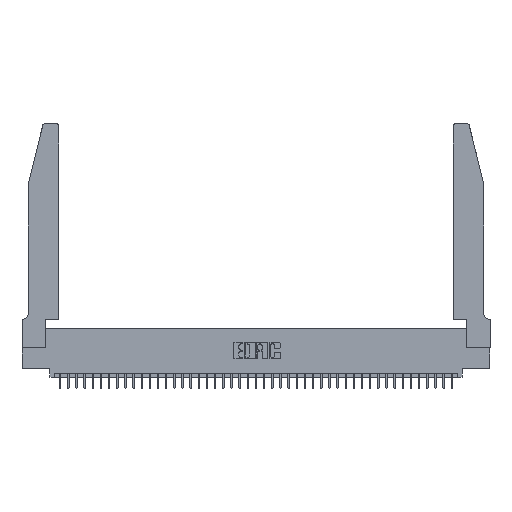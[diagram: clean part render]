
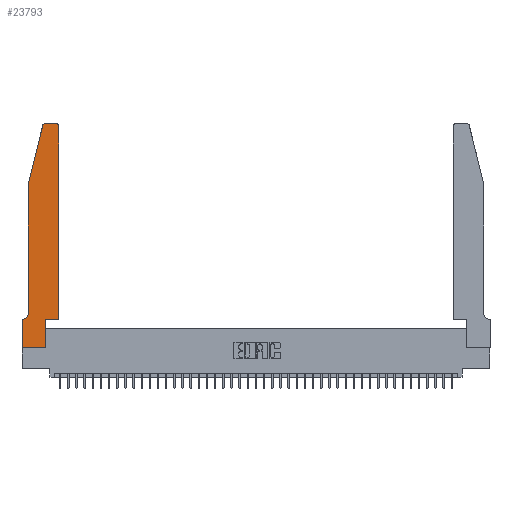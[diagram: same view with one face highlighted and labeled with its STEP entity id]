
A CAD part, top view. The second image highlights one B-rep face of the part: STEP entity #23793.
In plain terms, the highlighted planar face has unit normal (0, 0, 1).
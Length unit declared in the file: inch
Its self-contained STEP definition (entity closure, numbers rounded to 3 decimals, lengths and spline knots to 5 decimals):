
#125 = CARTESIAN_POINT ( 'NONE',  ( 0.0755, 2., 0.37 ) ) ;
#640 = CARTESIAN_POINT ( 'NONE',  ( 0.2865, 0., 0.37 ) ) ;
#813 = DIRECTION ( 'NONE',  ( 0., 1., 0. ) ) ;
#933 = CARTESIAN_POINT ( 'NONE',  ( 0.4505, 2.72, 0.37 ) ) ;
#1001 = FACE_OUTER_BOUND ( 'NONE', #10282, .T. ) ;
#1074 = CARTESIAN_POINT ( 'NONE',  ( 0.0055, 0.42, 0.37 ) ) ;
#1399 = VECTOR ( 'NONE', #2225, 39.37008 ) ;
#1448 = ORIENTED_EDGE ( 'NONE', *, *, #31188, .T. ) ;
#1595 = VERTEX_POINT ( 'NONE', #39212 ) ;
#1609 = VERTEX_POINT ( 'NONE', #39432 ) ;
#1884 = LINE ( 'NONE', #15031, #37617 ) ;
#1894 = VERTEX_POINT ( 'NONE', #22628 ) ;
#2225 = DIRECTION ( 'NONE',  ( 1., 0., 0. ) ) ;
#2980 = VERTEX_POINT ( 'NONE', #37067 ) ;
#3572 = DIRECTION ( 'NONE',  ( 0., 0., 1. ) ) ;
#4015 = CARTESIAN_POINT ( 'NONE',  ( 0.4505, 0.35, 0.37 ) ) ;
#5034 = CARTESIAN_POINT ( 'NONE',  ( 0., 0., 0.37 ) ) ;
#5152 = CIRCLE ( 'NONE', #27184, 0.03 ) ;
#6113 = VECTOR ( 'NONE', #37179, 39.37008 ) ;
#6641 = CIRCLE ( 'NONE', #32078, 0.07 ) ;
#6725 = ORIENTED_EDGE ( 'NONE', *, *, #13127, .T. ) ;
#6745 = EDGE_CURVE ( 'NONE', #12767, #1894, #1884, .T. ) ;
#7067 = LINE ( 'NONE', #27668, #12717 ) ;
#7109 = CARTESIAN_POINT ( 'NONE',  ( 0.284, 2.75, 0.37 ) ) ;
#7250 = ORIENTED_EDGE ( 'NONE', *, *, #20346, .T. ) ;
#7983 = EDGE_CURVE ( 'NONE', #29550, #2980, #7067, .T. ) ;
#8473 = DIRECTION ( 'NONE',  ( 1., 0., 0. ) ) ;
#8811 = DIRECTION ( 'NONE',  ( -1., 0., 0. ) ) ;
#9891 = DIRECTION ( 'NONE',  ( 0., 1., 0. ) ) ;
#10282 = EDGE_LOOP ( 'NONE', ( #7250, #13119, #25975, #40192, #32408, #32421, #6725, #27385, #17511, #1448, #28629, #17210 ) ) ;
#10356 = DIRECTION ( 'NONE',  ( 0., -1., 0. ) ) ;
#11438 = EDGE_CURVE ( 'NONE', #32144, #1609, #5152, .T. ) ;
#12012 = VERTEX_POINT ( 'NONE', #933 ) ;
#12025 = DIRECTION ( 'NONE',  ( 1., 0., 0. ) ) ;
#12665 = EDGE_CURVE ( 'NONE', #20466, #12012, #20432, .T. ) ;
#12717 = VECTOR ( 'NONE', #9891, 39.37008 ) ;
#12767 = VERTEX_POINT ( 'NONE', #125 ) ;
#13059 = DIRECTION ( 'NONE',  ( 1., 0., 0. ) ) ;
#13119 = ORIENTED_EDGE ( 'NONE', *, *, #11438, .T. ) ;
#13127 = EDGE_CURVE ( 'NONE', #22375, #37348, #19497, .T. ) ;
#13271 = CARTESIAN_POINT ( 'NONE',  ( 0.284, 2.72, 0.37 ) ) ;
#13286 = EDGE_CURVE ( 'NONE', #1894, #36201, #6641, .T. ) ;
#14137 = PLANE ( 'NONE',  #34084 ) ;
#14372 = DIRECTION ( 'NONE',  ( 0., -1., 0. ) ) ;
#15031 = CARTESIAN_POINT ( 'NONE',  ( 0.0755, 2., 0.37 ) ) ;
#15354 = LINE ( 'NONE', #25723, #42194 ) ;
#15478 = EDGE_CURVE ( 'NONE', #37348, #29550, #25954, .T. ) ;
#17210 = ORIENTED_EDGE ( 'NONE', *, *, #37333, .T. ) ;
#17251 = CARTESIAN_POINT ( 'NONE',  ( 0., 0., 0.37 ) ) ;
#17511 = ORIENTED_EDGE ( 'NONE', *, *, #7983, .T. ) ;
#18705 = CARTESIAN_POINT ( 'NONE',  ( 0.0755, 2., 0.37 ) ) ;
#19497 = LINE ( 'NONE', #17251, #34823 ) ;
#20346 = EDGE_CURVE ( 'NONE', #1595, #32144, #15354, .T. ) ;
#20432 = LINE ( 'NONE', #4015, #37236 ) ;
#20466 = VERTEX_POINT ( 'NONE', #23278 ) ;
#20826 = CARTESIAN_POINT ( 'NONE',  ( 0., 0.35, 0.37 ) ) ;
#21538 = CARTESIAN_POINT ( 'NONE',  ( 0.4505, 0.35, 0.37 ) ) ;
#21931 = LINE ( 'NONE', #18705, #40265 ) ;
#22069 = CARTESIAN_POINT ( 'NONE',  ( 0.4205, 2.72, 0.37 ) ) ;
#22109 = CARTESIAN_POINT ( 'NONE',  ( 0.0055, 0.35, 0.37 ) ) ;
#22375 = VERTEX_POINT ( 'NONE', #20826 ) ;
#22628 = CARTESIAN_POINT ( 'NONE',  ( 0.0755, 0.42, 0.37 ) ) ;
#23224 = AXIS2_PLACEMENT_3D ( 'NONE', #22069, #35205, #8473 ) ;
#23278 = CARTESIAN_POINT ( 'NONE',  ( 0.4505, 0.35, 0.37 ) ) ;
#23793 = ADVANCED_FACE ( 'NONE', ( #1001 ), #14137, .T. ) ;
#23888 = CIRCLE ( 'NONE', #23224, 0.03 ) ;
#24258 = DIRECTION ( 'NONE',  ( 0., 0., 1. ) ) ;
#24416 = EDGE_CURVE ( 'NONE', #1609, #12767, #21931, .T. ) ;
#25723 = CARTESIAN_POINT ( 'NONE',  ( 0.2605, 2.75, 0.37 ) ) ;
#25954 = LINE ( 'NONE', #39011, #1399 ) ;
#25975 = ORIENTED_EDGE ( 'NONE', *, *, #24416, .T. ) ;
#27184 = AXIS2_PLACEMENT_3D ( 'NONE', #13271, #3572, #13059 ) ;
#27385 = ORIENTED_EDGE ( 'NONE', *, *, #15478, .T. ) ;
#27503 = CARTESIAN_POINT ( 'NONE',  ( 0.0755, 0.35, 0.37 ) ) ;
#27668 = CARTESIAN_POINT ( 'NONE',  ( 0.2865, 0.35, 0.37 ) ) ;
#28629 = ORIENTED_EDGE ( 'NONE', *, *, #12665, .T. ) ;
#29550 = VERTEX_POINT ( 'NONE', #640 ) ;
#30912 = LINE ( 'NONE', #27503, #6113 ) ;
#30972 = LINE ( 'NONE', #21538, #31927 ) ;
#31188 = EDGE_CURVE ( 'NONE', #2980, #20466, #30972, .T. ) ;
#31801 = DIRECTION ( 'NONE',  ( -0.239, -0.971, 0. ) ) ;
#31927 = VECTOR ( 'NONE', #12025, 39.37008 ) ;
#32078 = AXIS2_PLACEMENT_3D ( 'NONE', #1074, #40453, #8811 ) ;
#32144 = VERTEX_POINT ( 'NONE', #7109 ) ;
#32408 = ORIENTED_EDGE ( 'NONE', *, *, #13286, .T. ) ;
#32421 = ORIENTED_EDGE ( 'NONE', *, *, #40711, .T. ) ;
#34084 = AXIS2_PLACEMENT_3D ( 'NONE', #40599, #24258, #41436 ) ;
#34823 = VECTOR ( 'NONE', #10356, 39.37008 ) ;
#35205 = DIRECTION ( 'NONE',  ( 0., 0., 1. ) ) ;
#36201 = VERTEX_POINT ( 'NONE', #22109 ) ;
#37067 = CARTESIAN_POINT ( 'NONE',  ( 0.2865, 0.35, 0.37 ) ) ;
#37179 = DIRECTION ( 'NONE',  ( -1., 0., 0. ) ) ;
#37236 = VECTOR ( 'NONE', #813, 39.37008 ) ;
#37333 = EDGE_CURVE ( 'NONE', #12012, #1595, #23888, .T. ) ;
#37348 = VERTEX_POINT ( 'NONE', #5034 ) ;
#37617 = VECTOR ( 'NONE', #14372, 39.37008 ) ;
#38769 = DIRECTION ( 'NONE',  ( -1., 0., 0. ) ) ;
#39011 = CARTESIAN_POINT ( 'NONE',  ( 0., 0., 0.37 ) ) ;
#39212 = CARTESIAN_POINT ( 'NONE',  ( 0.4205, 2.75, 0.37 ) ) ;
#39432 = CARTESIAN_POINT ( 'NONE',  ( 0.25487, 2.72718, 0.37 ) ) ;
#40192 = ORIENTED_EDGE ( 'NONE', *, *, #6745, .T. ) ;
#40265 = VECTOR ( 'NONE', #31801, 39.37008 ) ;
#40453 = DIRECTION ( 'NONE',  ( 0., 0., -1. ) ) ;
#40599 = CARTESIAN_POINT ( 'NONE',  ( 0., 0.35, 0.37 ) ) ;
#40711 = EDGE_CURVE ( 'NONE', #36201, #22375, #30912, .T. ) ;
#41436 = DIRECTION ( 'NONE',  ( 1., 0., 0. ) ) ;
#42194 = VECTOR ( 'NONE', #38769, 39.37008 ) ;
